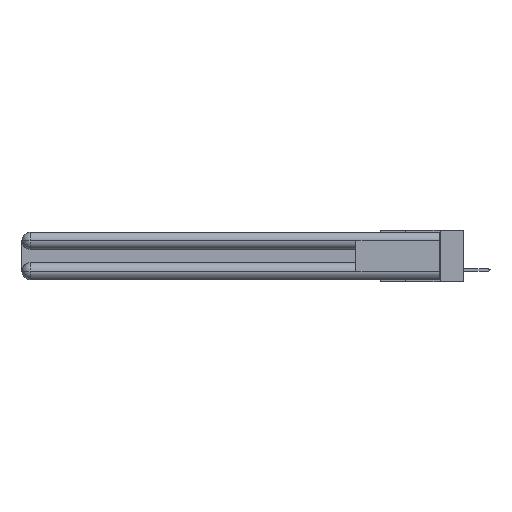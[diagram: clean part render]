
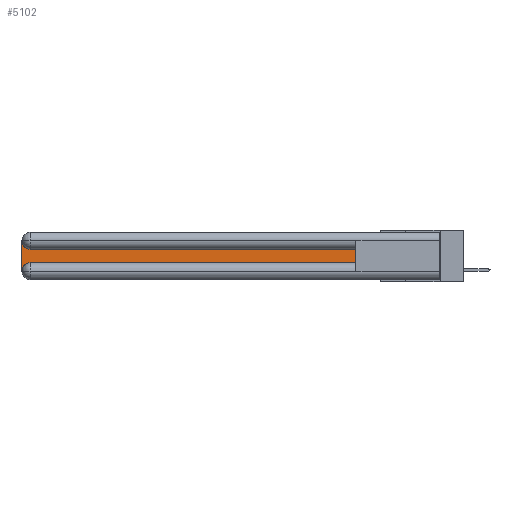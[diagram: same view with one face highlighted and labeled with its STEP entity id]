
A CAD part, left-side view. The second image highlights one B-rep face of the part: STEP entity #5102.
In plain terms, the highlighted planar face has unit normal (-1, 0, 0).
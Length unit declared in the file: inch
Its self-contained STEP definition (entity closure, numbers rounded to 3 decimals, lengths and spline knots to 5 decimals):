
#1579 = CARTESIAN_POINT ( 'NONE',  ( 0.075, 0.6, -0.1225 ) ) ;
#1724 = DIRECTION ( 'NONE',  ( 0., 0., 1. ) ) ;
#3828 = EDGE_CURVE ( 'NONE', #29789, #20317, #26986, .T. ) ;
#4590 = FACE_OUTER_BOUND ( 'NONE', #19801, .T. ) ;
#5102 = ADVANCED_FACE ( 'NONE', ( #4590 ), #6517, .F. ) ;
#6517 = PLANE ( 'NONE',  #16122 ) ;
#7170 = DIRECTION ( 'NONE',  ( 1., 0., 0. ) ) ;
#7283 = EDGE_CURVE ( 'NONE', #10642, #10537, #21999, .T. ) ;
#7448 = ORIENTED_EDGE ( 'NONE', *, *, #26330, .T. ) ;
#8877 = CARTESIAN_POINT ( 'NONE',  ( 0.075, 0.6, -0.2175 ) ) ;
#9011 = DIRECTION ( 'NONE',  ( 0., 0., -1. ) ) ;
#9339 = CARTESIAN_POINT ( 'NONE',  ( 0.075, 3., -0.0625 ) ) ;
#10078 = CARTESIAN_POINT ( 'NONE',  ( 0.075, 3., -0.2775 ) ) ;
#10537 = VERTEX_POINT ( 'NONE', #29037 ) ;
#10622 = CARTESIAN_POINT ( 'NONE',  ( 0.075, 3., -0.2175 ) ) ;
#10642 = VERTEX_POINT ( 'NONE', #19114 ) ;
#11111 = ORIENTED_EDGE ( 'NONE', *, *, #24992, .T. ) ;
#11199 = DIRECTION ( 'NONE',  ( 1., 0., 0. ) ) ;
#11537 = ORIENTED_EDGE ( 'NONE', *, *, #3828, .T. ) ;
#11732 = CARTESIAN_POINT ( 'NONE',  ( 0.075, 2.94, -0.2175 ) ) ;
#12187 = DIRECTION ( 'NONE',  ( 0., 0., -1. ) ) ;
#13289 = DIRECTION ( 'NONE',  ( 1., 0., 0. ) ) ;
#13968 = DIRECTION ( 'NONE',  ( 0., 1., 0. ) ) ;
#15043 = CARTESIAN_POINT ( 'NONE',  ( 0.075, 2.94, -0.0625 ) ) ;
#16122 = AXIS2_PLACEMENT_3D ( 'NONE', #26298, #11199, #9011 ) ;
#16248 = ORIENTED_EDGE ( 'NONE', *, *, #7283, .T. ) ;
#18655 = EDGE_CURVE ( 'NONE', #29894, #19775, #24797, .T. ) ;
#19114 = CARTESIAN_POINT ( 'NONE',  ( 0.075, 0.6, -0.1225 ) ) ;
#19775 = VERTEX_POINT ( 'NONE', #10078 ) ;
#19801 = EDGE_LOOP ( 'NONE', ( #16248, #22365, #19835, #7448, #11537, #11111 ) ) ;
#19835 = ORIENTED_EDGE ( 'NONE', *, *, #18655, .T. ) ;
#20317 = VERTEX_POINT ( 'NONE', #22926 ) ;
#21600 = VECTOR ( 'NONE', #13968, 39.37008 ) ;
#21999 = LINE ( 'NONE', #1579, #21600 ) ;
#22365 = ORIENTED_EDGE ( 'NONE', *, *, #31815, .T. ) ;
#22799 = DIRECTION ( 'NONE',  ( 0., 0., -1. ) ) ;
#22926 = CARTESIAN_POINT ( 'NONE',  ( 0.075, 0.6, -0.2175 ) ) ;
#23330 = DIRECTION ( 'NONE',  ( 0., 0., -1. ) ) ;
#23994 = VECTOR ( 'NONE', #22799, 39.37008 ) ;
#24416 = LINE ( 'NONE', #29178, #26413 ) ;
#24797 = LINE ( 'NONE', #10622, #23994 ) ;
#24992 = EDGE_CURVE ( 'NONE', #20317, #10642, #24416, .T. ) ;
#25091 = AXIS2_PLACEMENT_3D ( 'NONE', #30844, #13289, #23330 ) ;
#25109 = CIRCLE ( 'NONE', #25091, 0.06 ) ;
#25872 = CIRCLE ( 'NONE', #28360, 0.06 ) ;
#26298 = CARTESIAN_POINT ( 'NONE',  ( 0.075, 3., -0.1225 ) ) ;
#26330 = EDGE_CURVE ( 'NONE', #19775, #29789, #25109, .T. ) ;
#26413 = VECTOR ( 'NONE', #1724, 39.37008 ) ;
#26986 = LINE ( 'NONE', #8877, #30484 ) ;
#28360 = AXIS2_PLACEMENT_3D ( 'NONE', #15043, #7170, #12187 ) ;
#28570 = DIRECTION ( 'NONE',  ( 0., -1., 0. ) ) ;
#29037 = CARTESIAN_POINT ( 'NONE',  ( 0.075, 2.94, -0.1225 ) ) ;
#29178 = CARTESIAN_POINT ( 'NONE',  ( 0.075, 0.6, -0.2175 ) ) ;
#29789 = VERTEX_POINT ( 'NONE', #11732 ) ;
#29894 = VERTEX_POINT ( 'NONE', #9339 ) ;
#30484 = VECTOR ( 'NONE', #28570, 39.37008 ) ;
#30844 = CARTESIAN_POINT ( 'NONE',  ( 0.075, 2.94, -0.2775 ) ) ;
#31815 = EDGE_CURVE ( 'NONE', #10537, #29894, #25872, .T. ) ;
